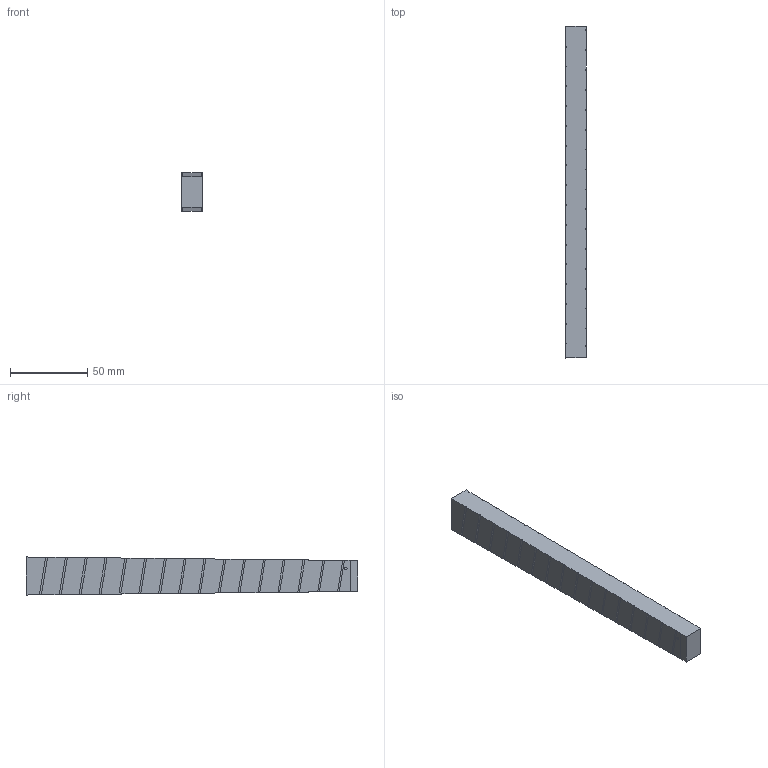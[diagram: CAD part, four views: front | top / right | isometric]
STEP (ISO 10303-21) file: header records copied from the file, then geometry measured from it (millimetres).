
FILE_DESCRIPTION(/* description */ (''),/* implementation_level */ '2;1');
FILE_NAME(/* name */ 'Middle Section.stp',/* time_stamp */ '2018-12-05T17:40:32-06:00',/* author */ ('johne'),/* organization */ (''),/* preprocessor_version */ 'ST-DEVELOPER v16.13',/* originating_system */ 'Autodesk Inventor 2018',/* authorisation */ '');
FILE_SCHEMA (('AUTOMOTIVE_DESIGN { 1 0 10303 214 3 1 1 }'));
Length unit declared in the file: millimetre
Products named in the file (1): Middle Section
Bounding box: 13.53 x 214.55 x 24.58 mm (x, y, z)
Volume: 63649.5 mm3; surface area: 16056.9 mm2
Topology: 1 solids, 1 shells, 81 faces, 242 edges, 162 vertices
Faces by surface type: bspline 41, plane 40
Entity records: 3517 total; most frequent: CARTESIAN_POINT 1386, ORIENTED_EDGE 484, DIRECTION 399, EDGE_CURVE 242, VERTEX_POINT 162, LINE 149, VECTOR 149, AXIS2_PLACEMENT_3D 125
